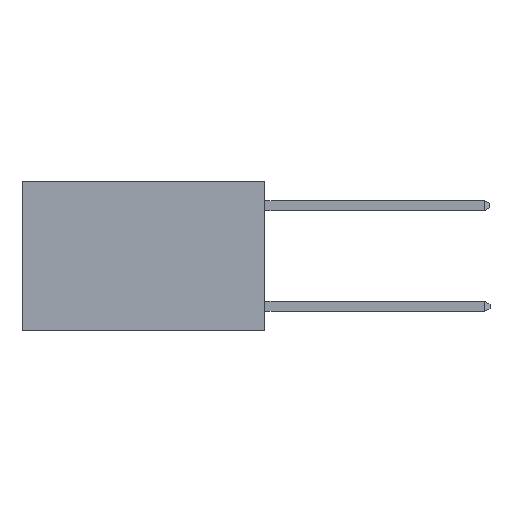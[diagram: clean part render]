
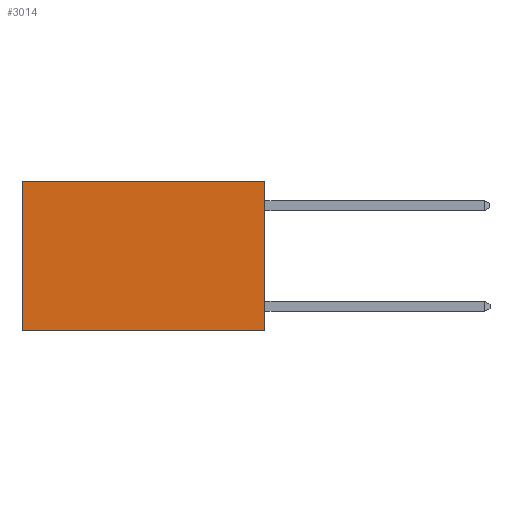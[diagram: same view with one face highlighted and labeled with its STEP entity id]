
A CAD part, left-side view. The second image highlights one B-rep face of the part: STEP entity #3014.
In plain terms, the highlighted planar face has unit normal (-1, 0, 0).
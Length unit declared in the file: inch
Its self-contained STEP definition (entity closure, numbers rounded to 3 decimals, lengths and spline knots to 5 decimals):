
#606 = CARTESIAN_POINT ( 'NONE',  ( 0.2625, 0.6, 0. ) ) ;
#662 = LINE ( 'NONE', #1857, #7382 ) ;
#852 = LINE ( 'NONE', #3110, #5884 ) ;
#1227 = DIRECTION ( 'NONE',  ( 0., 1., 0. ) ) ;
#1695 = VECTOR ( 'NONE', #5176, 39.37008 ) ;
#1788 = ORIENTED_EDGE ( 'NONE', *, *, #3282, .F. ) ;
#1857 = CARTESIAN_POINT ( 'NONE',  ( 0.2625, 0., -0.37 ) ) ;
#1976 = EDGE_CURVE ( 'NONE', #4629, #2438, #4280, .T. ) ;
#2212 = CARTESIAN_POINT ( 'NONE',  ( 0.2625, 0., 0. ) ) ;
#2438 = VERTEX_POINT ( 'NONE', #606 ) ;
#2515 = VECTOR ( 'NONE', #4074, 39.37008 ) ;
#2941 = CARTESIAN_POINT ( 'NONE',  ( 0.2625, 0., -0.37 ) ) ;
#3014 = ADVANCED_FACE ( 'NONE', ( #5211 ), #3739, .F. ) ;
#3110 = CARTESIAN_POINT ( 'NONE',  ( 0.2625, 0.6, 0. ) ) ;
#3163 = VERTEX_POINT ( 'NONE', #6970 ) ;
#3166 = EDGE_LOOP ( 'NONE', ( #5732, #4578, #1788, #8272 ) ) ;
#3282 = EDGE_CURVE ( 'NONE', #4629, #7283, #5009, .T. ) ;
#3727 = DIRECTION ( 'NONE',  ( 1., 0., 0. ) ) ;
#3739 = PLANE ( 'NONE',  #7140 ) ;
#3881 = DIRECTION ( 'NONE',  ( 0., 0., -1. ) ) ;
#4074 = DIRECTION ( 'NONE',  ( 0., 1., 0. ) ) ;
#4170 = CARTESIAN_POINT ( 'NONE',  ( 0.2625, 0., 0. ) ) ;
#4280 = LINE ( 'NONE', #4552, #2515 ) ;
#4552 = CARTESIAN_POINT ( 'NONE',  ( 0.2625, 0., 0. ) ) ;
#4578 = ORIENTED_EDGE ( 'NONE', *, *, #5943, .F. ) ;
#4629 = VERTEX_POINT ( 'NONE', #4170 ) ;
#5009 = LINE ( 'NONE', #6399, #1695 ) ;
#5148 = DIRECTION ( 'NONE',  ( 0., 0., -1. ) ) ;
#5176 = DIRECTION ( 'NONE',  ( 0., 0., -1. ) ) ;
#5211 = FACE_OUTER_BOUND ( 'NONE', #3166, .T. ) ;
#5732 = ORIENTED_EDGE ( 'NONE', *, *, #7474, .T. ) ;
#5884 = VECTOR ( 'NONE', #5148, 39.37008 ) ;
#5943 = EDGE_CURVE ( 'NONE', #7283, #3163, #662, .T. ) ;
#6399 = CARTESIAN_POINT ( 'NONE',  ( 0.2625, 0., 0. ) ) ;
#6970 = CARTESIAN_POINT ( 'NONE',  ( 0.2625, 0.6, -0.37 ) ) ;
#7140 = AXIS2_PLACEMENT_3D ( 'NONE', #2212, #3727, #3881 ) ;
#7283 = VERTEX_POINT ( 'NONE', #2941 ) ;
#7382 = VECTOR ( 'NONE', #1227, 39.37008 ) ;
#7474 = EDGE_CURVE ( 'NONE', #2438, #3163, #852, .T. ) ;
#8272 = ORIENTED_EDGE ( 'NONE', *, *, #1976, .T. ) ;
